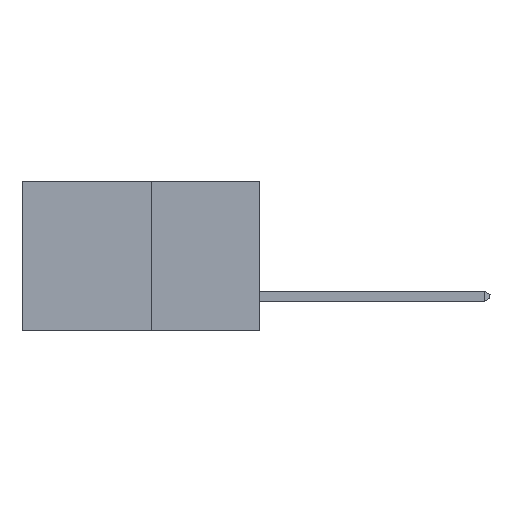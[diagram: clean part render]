
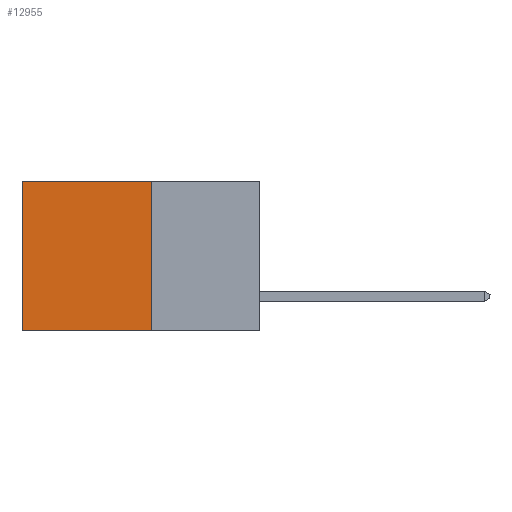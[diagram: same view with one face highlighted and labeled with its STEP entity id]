
A CAD part, left-side view. The second image highlights one B-rep face of the part: STEP entity #12955.
In plain terms, the highlighted planar face has unit normal (-1, 0, 0).
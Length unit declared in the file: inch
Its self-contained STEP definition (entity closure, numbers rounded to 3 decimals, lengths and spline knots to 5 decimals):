
#3216 = LINE ( 'NONE', #16578, #20405 ) ;
#4415 = EDGE_CURVE ( 'NONE', #10846, #5837, #3216, .T. ) ;
#4460 = CARTESIAN_POINT ( 'NONE',  ( 0.277, 0.59, -0.37 ) ) ;
#4994 = LINE ( 'NONE', #26915, #22190 ) ;
#5163 = ORIENTED_EDGE ( 'NONE', *, *, #9528, .F. ) ;
#5837 = VERTEX_POINT ( 'NONE', #8126 ) ;
#6773 = DIRECTION ( 'NONE',  ( 0., 0., -1. ) ) ;
#7355 = DIRECTION ( 'NONE',  ( 1., 0., 0. ) ) ;
#8126 = CARTESIAN_POINT ( 'NONE',  ( 0.277, 0.59, 0. ) ) ;
#9072 = LINE ( 'NONE', #23968, #20251 ) ;
#9528 = EDGE_CURVE ( 'NONE', #10846, #24855, #4994, .T. ) ;
#10846 = VERTEX_POINT ( 'NONE', #24579 ) ;
#11714 = CARTESIAN_POINT ( 'NONE',  ( 0.277, 0.27, -0.37 ) ) ;
#12955 = ADVANCED_FACE ( 'NONE', ( #20553 ), #18349, .F. ) ;
#15037 = DIRECTION ( 'NONE',  ( 0., 1., 0. ) ) ;
#16472 = DIRECTION ( 'NONE',  ( 0., 1., 0. ) ) ;
#16578 = CARTESIAN_POINT ( 'NONE',  ( 0.277, 0.27, 0. ) ) ;
#16706 = VERTEX_POINT ( 'NONE', #27614 ) ;
#16929 = EDGE_CURVE ( 'NONE', #24855, #16706, #9072, .T. ) ;
#17080 = EDGE_CURVE ( 'NONE', #5837, #16706, #18103, .T. ) ;
#18103 = LINE ( 'NONE', #4460, #27972 ) ;
#18349 = PLANE ( 'NONE',  #22584 ) ;
#20251 = VECTOR ( 'NONE', #15037, 39.37008 ) ;
#20405 = VECTOR ( 'NONE', #16472, 39.37008 ) ;
#20553 = FACE_OUTER_BOUND ( 'NONE', #22437, .T. ) ;
#20840 = ORIENTED_EDGE ( 'NONE', *, *, #17080, .T. ) ;
#22190 = VECTOR ( 'NONE', #22689, 39.37008 ) ;
#22437 = EDGE_LOOP ( 'NONE', ( #20840, #26141, #5163, #23123 ) ) ;
#22584 = AXIS2_PLACEMENT_3D ( 'NONE', #11714, #7355, #22991 ) ;
#22689 = DIRECTION ( 'NONE',  ( 0., 0., -1. ) ) ;
#22991 = DIRECTION ( 'NONE',  ( 0., 0., -1. ) ) ;
#23123 = ORIENTED_EDGE ( 'NONE', *, *, #4415, .T. ) ;
#23968 = CARTESIAN_POINT ( 'NONE',  ( 0.277, 0.27, -0.37 ) ) ;
#24579 = CARTESIAN_POINT ( 'NONE',  ( 0.277, 0.27, 0. ) ) ;
#24855 = VERTEX_POINT ( 'NONE', #28787 ) ;
#26141 = ORIENTED_EDGE ( 'NONE', *, *, #16929, .F. ) ;
#26915 = CARTESIAN_POINT ( 'NONE',  ( 0.277, 0.27, -0.37 ) ) ;
#27614 = CARTESIAN_POINT ( 'NONE',  ( 0.277, 0.59, -0.37 ) ) ;
#27972 = VECTOR ( 'NONE', #6773, 39.37008 ) ;
#28787 = CARTESIAN_POINT ( 'NONE',  ( 0.277, 0.27, -0.37 ) ) ;
